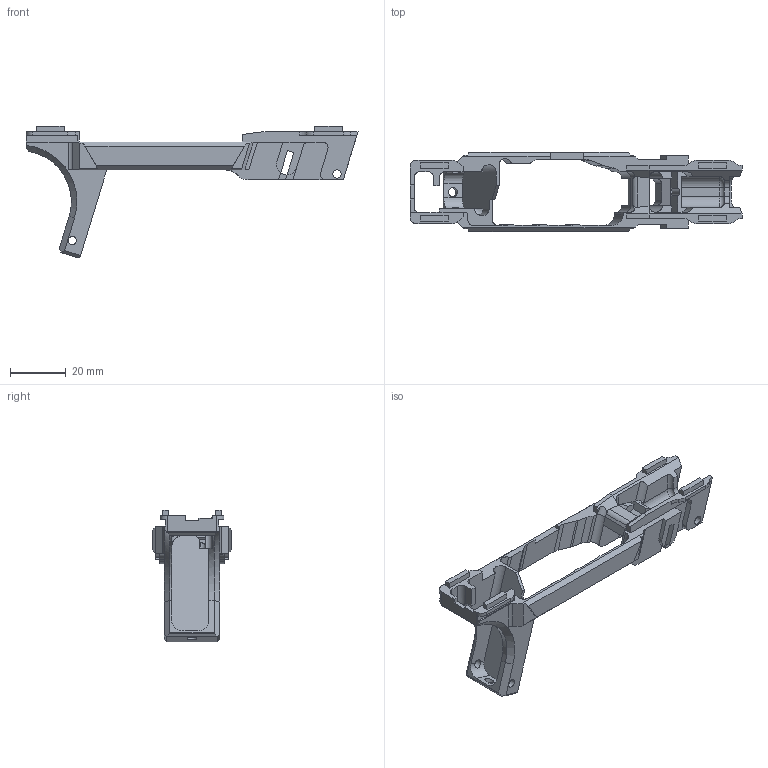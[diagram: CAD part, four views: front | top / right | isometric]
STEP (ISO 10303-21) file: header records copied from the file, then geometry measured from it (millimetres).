
FILE_DESCRIPTION(/* description */ (''),/* implementation_level */ '2;1');
FILE_NAME(/* name */ '120R REVH 80 Percent v4 v1.step',/* time_stamp */ '2025-07-25T11:31:31-05:00',/* author */ (''),/* organization */ (''),/* preprocessor_version */ 'ST-DEVELOPER v20.1',/* originating_system */ 'Autodesk Translation Framework v14.10.0.0',/* authorisation */ '');
FILE_SCHEMA (('AUTOMOTIVE_DESIGN { 1 0 10303 214 3 1 1 }'));
Length unit declared in the file: inch
Products named in the file (1): 120R REVH 80 Percent
Bounding box: 119 x 28.5 x 47.3 mm (x, y, z)
Volume: 15031.2 mm3; surface area: 12909.1 mm2
Topology: 1 solids, 1 shells, 288 faces, 846 edges, 550 vertices
Faces by surface type: plane 184, cylinder 96, cone 4, torus 2, bspline 2
Full cylindrical faces by diameter (mm): 3 x3, 3.175 x1, 3.332 x1
Entity records: 9730 total; most frequent: CARTESIAN_POINT 1873, ORIENTED_EDGE 1688, DIRECTION 1607, EDGE_CURVE 844, LINE 609, VECTOR 609, VERTEX_POINT 550, AXIS2_PLACEMENT_3D 499
